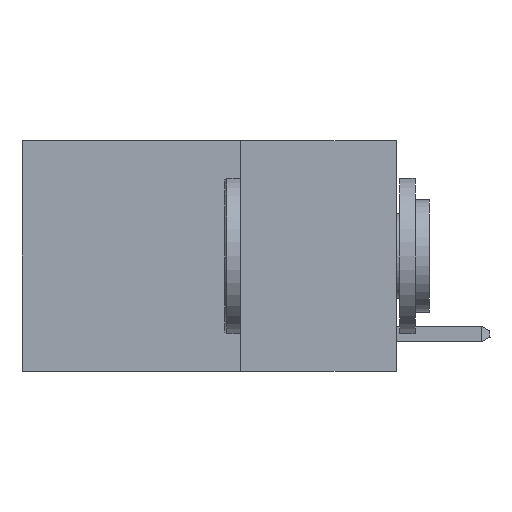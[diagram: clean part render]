
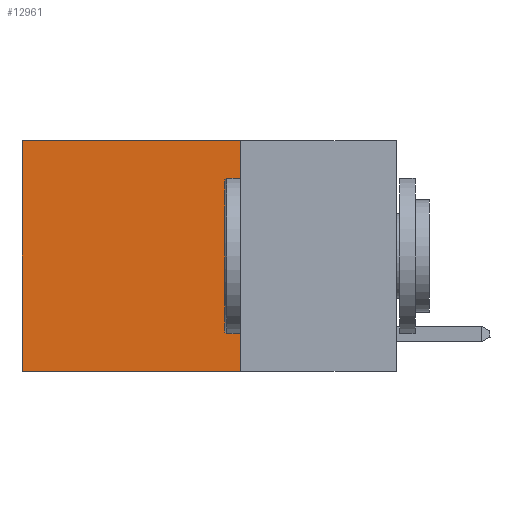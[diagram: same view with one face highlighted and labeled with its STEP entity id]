
A CAD part, left-side view. The second image highlights one B-rep face of the part: STEP entity #12961.
In plain terms, the highlighted planar face has unit normal (-1, 0, 0).
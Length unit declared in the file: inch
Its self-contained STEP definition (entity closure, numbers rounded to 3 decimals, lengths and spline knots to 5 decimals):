
#510 = EDGE_LOOP ( 'NONE', ( #18087, #10770, #14009, #18400 ) ) ;
#1326 = DIRECTION ( 'NONE',  ( 0., 1., 0. ) ) ;
#1414 = DIRECTION ( 'NONE',  ( 0., 0., -1. ) ) ;
#1848 = CARTESIAN_POINT ( 'NONE',  ( 0.2625, 0.25, 0. ) ) ;
#2356 = CARTESIAN_POINT ( 'NONE',  ( 0.2625, 0.25, 0. ) ) ;
#3105 = AXIS2_PLACEMENT_3D ( 'NONE', #2356, #13471, #3970 ) ;
#3411 = CARTESIAN_POINT ( 'NONE',  ( 0.2625, 0.6, 0. ) ) ;
#3970 = DIRECTION ( 'NONE',  ( 0., 0., -1. ) ) ;
#4905 = VERTEX_POINT ( 'NONE', #6907 ) ;
#5401 = VECTOR ( 'NONE', #1326, 39.37008 ) ;
#5755 = EDGE_CURVE ( 'NONE', #15403, #16552, #13797, .T. ) ;
#5891 = VECTOR ( 'NONE', #13577, 39.37008 ) ;
#6859 = EDGE_CURVE ( 'NONE', #16552, #13028, #10082, .T. ) ;
#6907 = CARTESIAN_POINT ( 'NONE',  ( 0.2625, 0.25, -0.37 ) ) ;
#7325 = CARTESIAN_POINT ( 'NONE',  ( 0.2625, 0.6, -0.37 ) ) ;
#10082 = LINE ( 'NONE', #10467, #5891 ) ;
#10266 = PLANE ( 'NONE',  #3105 ) ;
#10467 = CARTESIAN_POINT ( 'NONE',  ( 0.2625, 0.6, 0. ) ) ;
#10770 = ORIENTED_EDGE ( 'NONE', *, *, #15060, .F. ) ;
#11932 = EDGE_CURVE ( 'NONE', #15403, #4905, #20414, .T. ) ;
#12961 = ADVANCED_FACE ( 'NONE', ( #18239 ), #10266, .F. ) ;
#13028 = VERTEX_POINT ( 'NONE', #7325 ) ;
#13471 = DIRECTION ( 'NONE',  ( 1., 0., 0. ) ) ;
#13577 = DIRECTION ( 'NONE',  ( 0., 0., -1. ) ) ;
#13797 = LINE ( 'NONE', #20198, #5401 ) ;
#14009 = ORIENTED_EDGE ( 'NONE', *, *, #11932, .F. ) ;
#15060 = EDGE_CURVE ( 'NONE', #4905, #13028, #20310, .T. ) ;
#15209 = CARTESIAN_POINT ( 'NONE',  ( 0.2625, 0.25, -0.37 ) ) ;
#15403 = VERTEX_POINT ( 'NONE', #1848 ) ;
#16276 = VECTOR ( 'NONE', #1414, 39.37008 ) ;
#16552 = VERTEX_POINT ( 'NONE', #3411 ) ;
#16784 = DIRECTION ( 'NONE',  ( 0., 1., 0. ) ) ;
#18087 = ORIENTED_EDGE ( 'NONE', *, *, #6859, .T. ) ;
#18239 = FACE_OUTER_BOUND ( 'NONE', #510, .T. ) ;
#18400 = ORIENTED_EDGE ( 'NONE', *, *, #5755, .T. ) ;
#18737 = CARTESIAN_POINT ( 'NONE',  ( 0.2625, 0.25, 0. ) ) ;
#19817 = VECTOR ( 'NONE', #16784, 39.37008 ) ;
#20198 = CARTESIAN_POINT ( 'NONE',  ( 0.2625, 0.25, 0. ) ) ;
#20310 = LINE ( 'NONE', #15209, #19817 ) ;
#20414 = LINE ( 'NONE', #18737, #16276 ) ;
